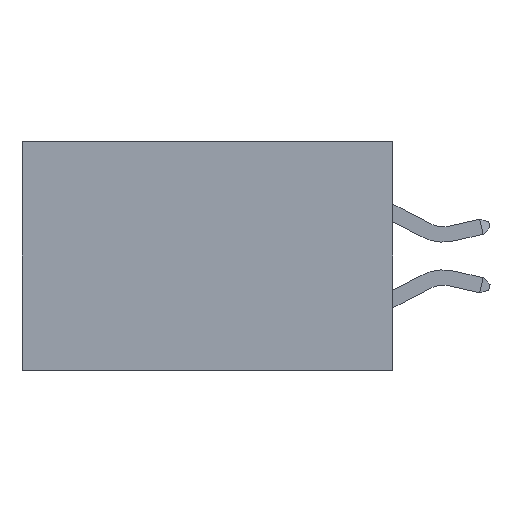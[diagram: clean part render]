
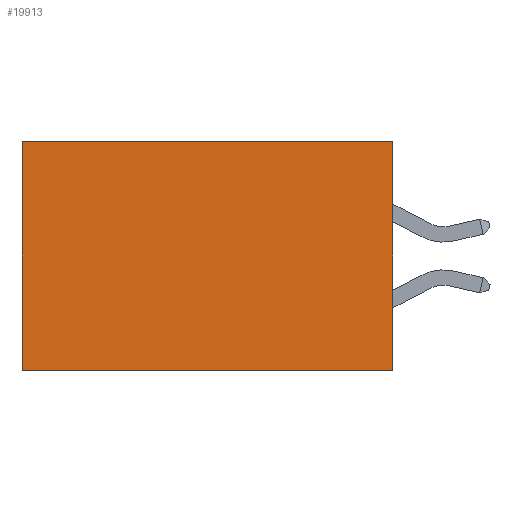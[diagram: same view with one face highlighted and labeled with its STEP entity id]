
A CAD part, left-side view. The second image highlights one B-rep face of the part: STEP entity #19913.
In plain terms, the highlighted planar face has unit normal (-1, 0, 0).
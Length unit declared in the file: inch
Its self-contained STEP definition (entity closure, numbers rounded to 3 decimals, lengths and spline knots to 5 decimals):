
#20 = CARTESIAN_POINT ( 'NONE',  ( 0.2875, 0.6, 0. ) ) ;
#233 = CARTESIAN_POINT ( 'NONE',  ( 0.2875, 0.6, 0. ) ) ;
#2087 = VECTOR ( 'NONE', #16900, 39.37008 ) ;
#2317 = EDGE_CURVE ( 'NONE', #7885, #11680, #10144, .T. ) ;
#2831 = VERTEX_POINT ( 'NONE', #11202 ) ;
#3694 = DIRECTION ( 'NONE',  ( 0., 1., 0. ) ) ;
#4063 = DIRECTION ( 'NONE',  ( 1., 0., 0. ) ) ;
#5630 = DIRECTION ( 'NONE',  ( 0., 0., -1. ) ) ;
#5664 = DIRECTION ( 'NONE',  ( 0., 0., -1. ) ) ;
#6561 = LINE ( 'NONE', #10006, #10187 ) ;
#6695 = DIRECTION ( 'NONE',  ( 0., 0., -1. ) ) ;
#7803 = CARTESIAN_POINT ( 'NONE',  ( 0.2875, 0., 0. ) ) ;
#7885 = VERTEX_POINT ( 'NONE', #17574 ) ;
#7990 = CARTESIAN_POINT ( 'NONE',  ( 0.2875, 0., 0. ) ) ;
#8701 = CARTESIAN_POINT ( 'NONE',  ( 0.2875, 0., 0. ) ) ;
#9130 = LINE ( 'NONE', #7803, #2087 ) ;
#9365 = AXIS2_PLACEMENT_3D ( 'NONE', #8701, #4063, #5630 ) ;
#10006 = CARTESIAN_POINT ( 'NONE',  ( 0.2875, 0., -0.37 ) ) ;
#10144 = LINE ( 'NONE', #7990, #14704 ) ;
#10187 = VECTOR ( 'NONE', #3694, 39.37008 ) ;
#11202 = CARTESIAN_POINT ( 'NONE',  ( 0.2875, 0.6, -0.37 ) ) ;
#11630 = VERTEX_POINT ( 'NONE', #233 ) ;
#11680 = VERTEX_POINT ( 'NONE', #15661 ) ;
#11783 = EDGE_LOOP ( 'NONE', ( #16871, #17093, #18678, #17820 ) ) ;
#13252 = EDGE_CURVE ( 'NONE', #11680, #2831, #6561, .T. ) ;
#14704 = VECTOR ( 'NONE', #5664, 39.37008 ) ;
#14889 = LINE ( 'NONE', #20, #16582 ) ;
#15047 = EDGE_CURVE ( 'NONE', #7885, #11630, #9130, .T. ) ;
#15661 = CARTESIAN_POINT ( 'NONE',  ( 0.2875, 0., -0.37 ) ) ;
#15866 = FACE_OUTER_BOUND ( 'NONE', #11783, .T. ) ;
#16582 = VECTOR ( 'NONE', #6695, 39.37008 ) ;
#16871 = ORIENTED_EDGE ( 'NONE', *, *, #19755, .T. ) ;
#16900 = DIRECTION ( 'NONE',  ( 0., 1., 0. ) ) ;
#17093 = ORIENTED_EDGE ( 'NONE', *, *, #13252, .F. ) ;
#17574 = CARTESIAN_POINT ( 'NONE',  ( 0.2875, 0., 0. ) ) ;
#17820 = ORIENTED_EDGE ( 'NONE', *, *, #15047, .T. ) ;
#18678 = ORIENTED_EDGE ( 'NONE', *, *, #2317, .F. ) ;
#19441 = PLANE ( 'NONE',  #9365 ) ;
#19755 = EDGE_CURVE ( 'NONE', #11630, #2831, #14889, .T. ) ;
#19913 = ADVANCED_FACE ( 'NONE', ( #15866 ), #19441, .F. ) ;
